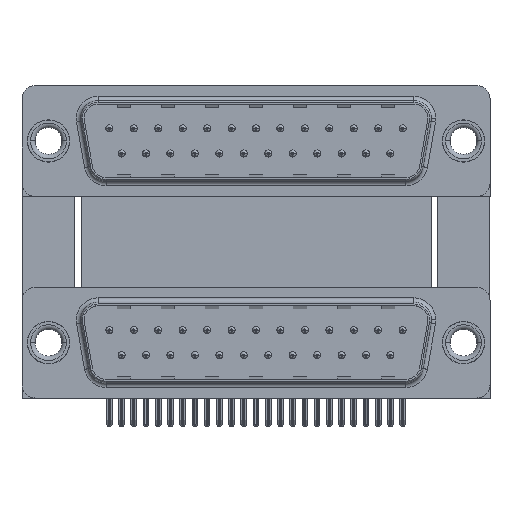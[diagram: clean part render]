
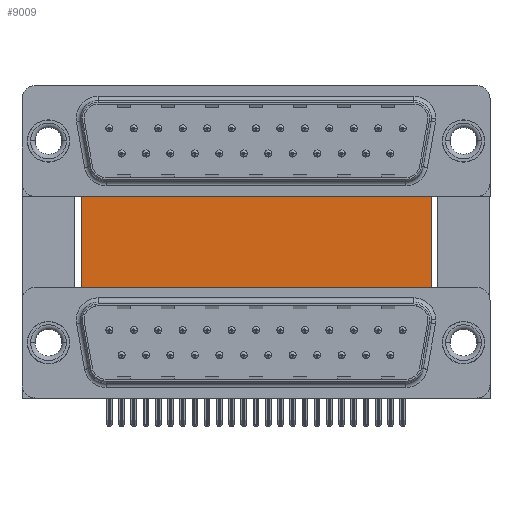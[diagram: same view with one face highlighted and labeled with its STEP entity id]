
A CAD part, top view. The second image highlights one B-rep face of the part: STEP entity #9009.
In plain terms, the highlighted planar face has unit normal (0, 0, 1).
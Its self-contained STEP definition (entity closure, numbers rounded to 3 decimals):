
#37 = DIRECTION ( 'NONE',  ( 0., -1., 0. ) ) ;
#1585 = PLANE ( 'NONE',  #26724 ) ;
#4118 = DIRECTION ( 'NONE',  ( 1., 0., 0. ) ) ;
#5060 = CARTESIAN_POINT ( 'NONE',  ( 3.79, 16.585, -12. ) ) ;
#9009 = ADVANCED_FACE ( 'NONE', ( #17707 ), #1585, .F. ) ;
#9093 = ORIENTED_EDGE ( 'NONE', *, *, #17730, .F. ) ;
#9759 = EDGE_LOOP ( 'NONE', ( #26095, #9093, #37953, #27308 ) ) ;
#10048 = VECTOR ( 'NONE', #37, 1000. ) ;
#12712 = VERTEX_POINT ( 'NONE', #14507 ) ;
#13750 = CARTESIAN_POINT ( 'NONE',  ( 3.79, 16.585, -12. ) ) ;
#14507 = CARTESIAN_POINT ( 'NONE',  ( 43.43, -3.735, -12. ) ) ;
#15227 = VECTOR ( 'NONE', #4118, 1000. ) ;
#15527 = VERTEX_POINT ( 'NONE', #13750 ) ;
#17373 = EDGE_CURVE ( 'NONE', #15527, #32923, #29244, .T. ) ;
#17707 = FACE_OUTER_BOUND ( 'NONE', #9759, .T. ) ;
#17730 = EDGE_CURVE ( 'NONE', #32923, #12712, #24947, .T. ) ;
#18019 = CARTESIAN_POINT ( 'NONE',  ( 43.43, 16.585, -12. ) ) ;
#18069 = VECTOR ( 'NONE', #24392, 1000. ) ;
#18426 = VECTOR ( 'NONE', #32900, 1000. ) ;
#20380 = DIRECTION ( 'NONE',  ( -1., 0., 0. ) ) ;
#20766 = CARTESIAN_POINT ( 'NONE',  ( 3.79, -3.735, -12. ) ) ;
#23500 = CARTESIAN_POINT ( 'NONE',  ( 3.79, 16.585, -12. ) ) ;
#24392 = DIRECTION ( 'NONE',  ( 1., 0., 0. ) ) ;
#24947 = LINE ( 'NONE', #18019, #10048 ) ;
#25011 = EDGE_CURVE ( 'NONE', #15527, #34165, #33104, .T. ) ;
#26095 = ORIENTED_EDGE ( 'NONE', *, *, #32139, .T. ) ;
#26507 = DIRECTION ( 'NONE',  ( 0., 0., -1. ) ) ;
#26724 = AXIS2_PLACEMENT_3D ( 'NONE', #5060, #26507, #20380 ) ;
#27308 = ORIENTED_EDGE ( 'NONE', *, *, #25011, .T. ) ;
#27465 = CARTESIAN_POINT ( 'NONE',  ( 3.79, -3.735, -12. ) ) ;
#29244 = LINE ( 'NONE', #32100, #15227 ) ;
#32100 = CARTESIAN_POINT ( 'NONE',  ( 3.79, 16.585, -12. ) ) ;
#32139 = EDGE_CURVE ( 'NONE', #34165, #12712, #40289, .T. ) ;
#32900 = DIRECTION ( 'NONE',  ( 0., -1., 0. ) ) ;
#32923 = VERTEX_POINT ( 'NONE', #36310 ) ;
#33104 = LINE ( 'NONE', #23500, #18426 ) ;
#34165 = VERTEX_POINT ( 'NONE', #20766 ) ;
#36310 = CARTESIAN_POINT ( 'NONE',  ( 43.43, 16.585, -12. ) ) ;
#37953 = ORIENTED_EDGE ( 'NONE', *, *, #17373, .F. ) ;
#40289 = LINE ( 'NONE', #27465, #18069 ) ;
